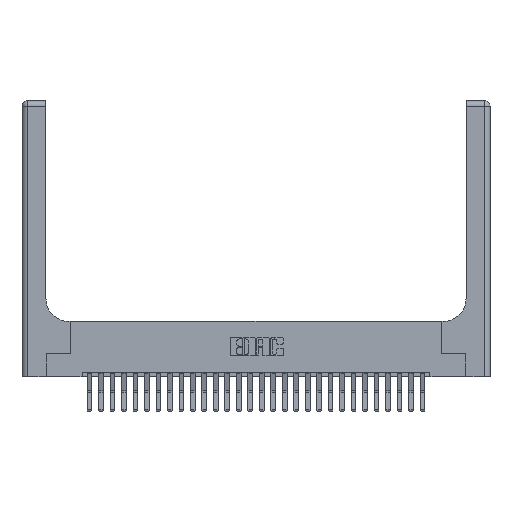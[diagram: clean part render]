
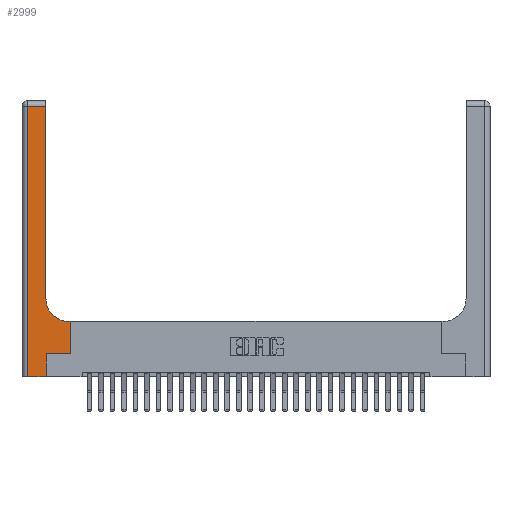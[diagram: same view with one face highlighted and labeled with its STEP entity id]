
A CAD part, top view. The second image highlights one B-rep face of the part: STEP entity #2999.
In plain terms, the highlighted planar face has unit normal (0, 0, 1).
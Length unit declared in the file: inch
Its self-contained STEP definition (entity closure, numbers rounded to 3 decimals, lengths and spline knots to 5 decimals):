
#398 = EDGE_CURVE ( 'NONE', #17088, #13566, #25249, .T. ) ;
#1108 = VERTEX_POINT ( 'NONE', #2427 ) ;
#1262 = CIRCLE ( 'NONE', #23025, 0.25 ) ;
#1721 = DIRECTION ( 'NONE',  ( 1., 0., 0. ) ) ;
#1970 = CARTESIAN_POINT ( 'NONE',  ( 0.265, 0., 0.37 ) ) ;
#2425 = CARTESIAN_POINT ( 'NONE',  ( 0.06, 0., 0.37 ) ) ;
#2427 = CARTESIAN_POINT ( 'NONE',  ( 0.265, 0.25, 0.37 ) ) ;
#2440 = VERTEX_POINT ( 'NONE', #17162 ) ;
#2675 = VECTOR ( 'NONE', #25446, 39.37008 ) ;
#2744 = EDGE_CURVE ( 'NONE', #21536, #5996, #20402, .T. ) ;
#2977 = VECTOR ( 'NONE', #8619, 39.37008 ) ;
#2999 = ADVANCED_FACE ( 'NONE', ( #11767 ), #20082, .F. ) ;
#3127 = LINE ( 'NONE', #5432, #4386 ) ;
#3670 = ORIENTED_EDGE ( 'NONE', *, *, #26144, .T. ) ;
#4386 = VECTOR ( 'NONE', #11166, 39.37008 ) ;
#4460 = VECTOR ( 'NONE', #1721, 39.37008 ) ;
#5102 = CARTESIAN_POINT ( 'NONE',  ( 0.265, 0., 0.37 ) ) ;
#5166 = ORIENTED_EDGE ( 'NONE', *, *, #2744, .T. ) ;
#5190 = VECTOR ( 'NONE', #6581, 39.37008 ) ;
#5432 = CARTESIAN_POINT ( 'NONE',  ( 0.06, 3., 0.37 ) ) ;
#5756 = EDGE_LOOP ( 'NONE', ( #20769, #25680, #8891, #5166, #12119, #3670, #16723, #12016, #17598 ) ) ;
#5768 = DIRECTION ( 'NONE',  ( 0., 0., -1. ) ) ;
#5996 = VERTEX_POINT ( 'NONE', #5102 ) ;
#6581 = DIRECTION ( 'NONE',  ( -1., 0., 0. ) ) ;
#7230 = CARTESIAN_POINT ( 'NONE',  ( 0.26, 2.94, 0.37 ) ) ;
#7401 = CARTESIAN_POINT ( 'NONE',  ( 0., 3., 0.37 ) ) ;
#7420 = VERTEX_POINT ( 'NONE', #12199 ) ;
#8589 = CARTESIAN_POINT ( 'NONE',  ( 0.06, 2.94, 0.37 ) ) ;
#8619 = DIRECTION ( 'NONE',  ( -1., 0., 0. ) ) ;
#8891 = ORIENTED_EDGE ( 'NONE', *, *, #11837, .T. ) ;
#9714 = DIRECTION ( 'NONE',  ( 0., 0., -1. ) ) ;
#9939 = VERTEX_POINT ( 'NONE', #23889 ) ;
#10314 = EDGE_CURVE ( 'NONE', #7420, #11353, #25247, .T. ) ;
#11166 = DIRECTION ( 'NONE',  ( 0., -1., 0. ) ) ;
#11353 = VERTEX_POINT ( 'NONE', #18481 ) ;
#11371 = EDGE_CURVE ( 'NONE', #5996, #1108, #24731, .T. ) ;
#11767 = FACE_OUTER_BOUND ( 'NONE', #5756, .T. ) ;
#11837 = EDGE_CURVE ( 'NONE', #13566, #21536, #3127, .T. ) ;
#11870 = AXIS2_PLACEMENT_3D ( 'NONE', #7401, #9714, #13802 ) ;
#12016 = ORIENTED_EDGE ( 'NONE', *, *, #10314, .T. ) ;
#12119 = ORIENTED_EDGE ( 'NONE', *, *, #11371, .T. ) ;
#12199 = CARTESIAN_POINT ( 'NONE',  ( 0.528, 0.6, 0.37 ) ) ;
#12250 = EDGE_CURVE ( 'NONE', #2440, #7420, #17150, .T. ) ;
#12429 = CARTESIAN_POINT ( 'NONE',  ( 0.51, 0.85, 0.37 ) ) ;
#12753 = DIRECTION ( 'NONE',  ( 0., 1., 0. ) ) ;
#13566 = VERTEX_POINT ( 'NONE', #8589 ) ;
#13802 = DIRECTION ( 'NONE',  ( -1., 0., 0. ) ) ;
#13933 = VECTOR ( 'NONE', #12753, 39.37008 ) ;
#15352 = DIRECTION ( 'NONE',  ( 1., 0., 0. ) ) ;
#15751 = LINE ( 'NONE', #17262, #25144 ) ;
#15780 = CARTESIAN_POINT ( 'NONE',  ( 0., 0., 0.37 ) ) ;
#16723 = ORIENTED_EDGE ( 'NONE', *, *, #12250, .T. ) ;
#17083 = CARTESIAN_POINT ( 'NONE',  ( 0.26, 0.6, 0.37 ) ) ;
#17088 = VERTEX_POINT ( 'NONE', #7230 ) ;
#17150 = LINE ( 'NONE', #23273, #2675 ) ;
#17162 = CARTESIAN_POINT ( 'NONE',  ( 0.528, 0.25, 0.37 ) ) ;
#17262 = CARTESIAN_POINT ( 'NONE',  ( 0.265, 0.25, 0.37 ) ) ;
#17598 = ORIENTED_EDGE ( 'NONE', *, *, #18089, .T. ) ;
#18089 = EDGE_CURVE ( 'NONE', #11353, #9939, #1262, .T. ) ;
#18141 = VECTOR ( 'NONE', #21599, 39.37008 ) ;
#18481 = CARTESIAN_POINT ( 'NONE',  ( 0.51, 0.6, 0.37 ) ) ;
#20082 = PLANE ( 'NONE',  #11870 ) ;
#20402 = LINE ( 'NONE', #15780, #4460 ) ;
#20769 = ORIENTED_EDGE ( 'NONE', *, *, #23616, .T. ) ;
#21536 = VERTEX_POINT ( 'NONE', #2425 ) ;
#21599 = DIRECTION ( 'NONE',  ( 0., 1., 0. ) ) ;
#21874 = CARTESIAN_POINT ( 'NONE',  ( 0.26, 3., 0.37 ) ) ;
#23025 = AXIS2_PLACEMENT_3D ( 'NONE', #12429, #5768, #24691 ) ;
#23273 = CARTESIAN_POINT ( 'NONE',  ( 0.528, 0.25, 0.37 ) ) ;
#23616 = EDGE_CURVE ( 'NONE', #9939, #17088, #23775, .T. ) ;
#23775 = LINE ( 'NONE', #21874, #18141 ) ;
#23889 = CARTESIAN_POINT ( 'NONE',  ( 0.26, 0.85, 0.37 ) ) ;
#24691 = DIRECTION ( 'NONE',  ( 1., 0., 0. ) ) ;
#24731 = LINE ( 'NONE', #1970, #13933 ) ;
#25103 = CARTESIAN_POINT ( 'NONE',  ( 0., 2.94, 0.37 ) ) ;
#25144 = VECTOR ( 'NONE', #15352, 39.37008 ) ;
#25247 = LINE ( 'NONE', #17083, #5190 ) ;
#25249 = LINE ( 'NONE', #25103, #2977 ) ;
#25446 = DIRECTION ( 'NONE',  ( 0., 1., 0. ) ) ;
#25680 = ORIENTED_EDGE ( 'NONE', *, *, #398, .T. ) ;
#26144 = EDGE_CURVE ( 'NONE', #1108, #2440, #15751, .T. ) ;
